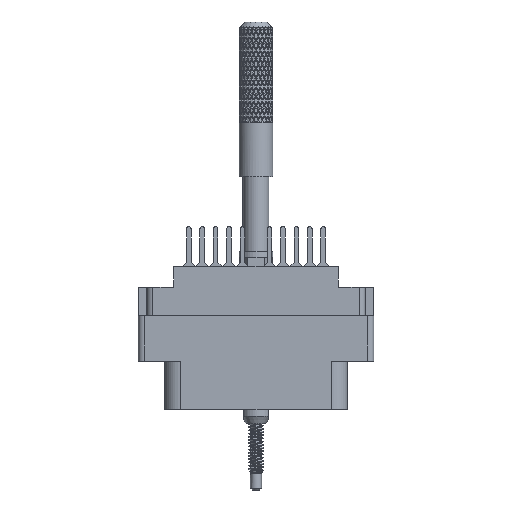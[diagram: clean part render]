
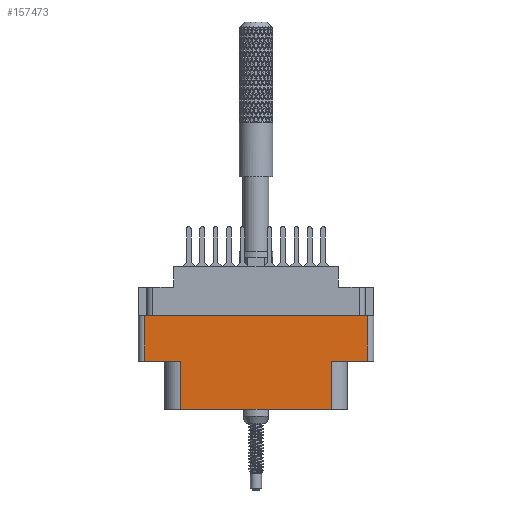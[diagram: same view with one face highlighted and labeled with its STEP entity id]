
A CAD part, front view. The second image highlights one B-rep face of the part: STEP entity #157473.
In plain terms, the highlighted planar face has unit normal (0, -1, 0).
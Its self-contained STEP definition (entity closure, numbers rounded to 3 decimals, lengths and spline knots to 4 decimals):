
#1881 = CARTESIAN_POINT ( 'NONE',  ( 0., -0.343, -0.529 ) ) ;
#3658 = LINE ( 'NONE', #1881, #130490 ) ;
#9122 = CARTESIAN_POINT ( 'NONE',  ( -0.656, -0.343, -0.798 ) ) ;
#9494 = LINE ( 'NONE', #136040, #165769 ) ;
#14220 = LINE ( 'NONE', #177238, #127639 ) ;
#16859 = ORIENTED_EDGE ( 'NONE', *, *, #94489, .T. ) ;
#19193 = EDGE_CURVE ( 'NONE', #113057, #141740, #3658, .T. ) ;
#19745 = CARTESIAN_POINT ( 'NONE',  ( -0.4205, -0.343, -0.798 ) ) ;
#21551 = ORIENTED_EDGE ( 'NONE', *, *, #19193, .F. ) ;
#22497 = CARTESIAN_POINT ( 'NONE',  ( -0.624, -0.343, -0.274 ) ) ;
#24329 = DIRECTION ( 'NONE',  ( 0., 0., -1. ) ) ;
#25174 = CARTESIAN_POINT ( 'NONE',  ( 0.4205, -0.343, -0.529 ) ) ;
#26134 = LINE ( 'NONE', #150712, #37382 ) ;
#28182 = DIRECTION ( 'NONE',  ( 1., 0., 0. ) ) ;
#31540 = EDGE_CURVE ( 'NONE', #138712, #152731, #26134, .T. ) ;
#34673 = DIRECTION ( 'NONE',  ( 1., 0., 0. ) ) ;
#36515 = VECTOR ( 'NONE', #28182, 39.3701 ) ;
#37382 = VECTOR ( 'NONE', #105849, 39.3701 ) ;
#37632 = VERTEX_POINT ( 'NONE', #130890 ) ;
#40398 = LINE ( 'NONE', #182762, #153810 ) ;
#48105 = VERTEX_POINT ( 'NONE', #68796 ) ;
#52549 = DIRECTION ( 'NONE',  ( 0., 0., 1. ) ) ;
#57459 = LINE ( 'NONE', #115490, #143591 ) ;
#58088 = DIRECTION ( 'NONE',  ( 0., 0., -1. ) ) ;
#60278 = VECTOR ( 'NONE', #52549, 39.3701 ) ;
#63743 = CARTESIAN_POINT ( 'NONE',  ( 0.624, -0.343, -0.274 ) ) ;
#67475 = DIRECTION ( 'NONE',  ( 0., -1., 0. ) ) ;
#68796 = CARTESIAN_POINT ( 'NONE',  ( 0.4205, -0.343, -0.798 ) ) ;
#71925 = ORIENTED_EDGE ( 'NONE', *, *, #114948, .T. ) ;
#73139 = EDGE_CURVE ( 'NONE', #152731, #37632, #75207, .T. ) ;
#74590 = ORIENTED_EDGE ( 'NONE', *, *, #175063, .T. ) ;
#75143 = ORIENTED_EDGE ( 'NONE', *, *, #117108, .F. ) ;
#75207 = LINE ( 'NONE', #102391, #36515 ) ;
#76199 = LINE ( 'NONE', #112153, #60278 ) ;
#81709 = VERTEX_POINT ( 'NONE', #63743 ) ;
#82576 = FACE_OUTER_BOUND ( 'NONE', #109421, .T. ) ;
#86881 = DIRECTION ( 'NONE',  ( -1., 0., 0. ) ) ;
#94489 = EDGE_CURVE ( 'NONE', #142063, #48105, #40398, .T. ) ;
#102391 = CARTESIAN_POINT ( 'NONE',  ( 0., -0.343, -0.529 ) ) ;
#105309 = ORIENTED_EDGE ( 'NONE', *, *, #73139, .T. ) ;
#105849 = DIRECTION ( 'NONE',  ( 0., 0., -1. ) ) ;
#109421 = EDGE_LOOP ( 'NONE', ( #75143, #126538, #105309, #71925, #16859, #113337, #21551, #74590 ) ) ;
#112153 = CARTESIAN_POINT ( 'NONE',  ( 0.4205, -0.343, -0.529 ) ) ;
#113057 = VERTEX_POINT ( 'NONE', #121428 ) ;
#113337 = ORIENTED_EDGE ( 'NONE', *, *, #127211, .T. ) ;
#114948 = EDGE_CURVE ( 'NONE', #37632, #142063, #14220, .T. ) ;
#115490 = CARTESIAN_POINT ( 'NONE',  ( 0.624, -0.343, -0.798 ) ) ;
#117108 = EDGE_CURVE ( 'NONE', #138712, #81709, #9494, .T. ) ;
#121428 = CARTESIAN_POINT ( 'NONE',  ( 0.624, -0.343, -0.529 ) ) ;
#125659 = PLANE ( 'NONE',  #184374 ) ;
#126538 = ORIENTED_EDGE ( 'NONE', *, *, #31540, .T. ) ;
#127211 = EDGE_CURVE ( 'NONE', #48105, #141740, #76199, .T. ) ;
#127639 = VECTOR ( 'NONE', #58088, 39.3701 ) ;
#128071 = DIRECTION ( 'NONE',  ( 1., 0., 0. ) ) ;
#130490 = VECTOR ( 'NONE', #86881, 39.3701 ) ;
#130890 = CARTESIAN_POINT ( 'NONE',  ( -0.4205, -0.343, -0.529 ) ) ;
#136040 = CARTESIAN_POINT ( 'NONE',  ( 0., -0.343, -0.274 ) ) ;
#138712 = VERTEX_POINT ( 'NONE', #22497 ) ;
#141740 = VERTEX_POINT ( 'NONE', #25174 ) ;
#142063 = VERTEX_POINT ( 'NONE', #19745 ) ;
#143591 = VECTOR ( 'NONE', #145784, 39.3701 ) ;
#145784 = DIRECTION ( 'NONE',  ( 0., 0., 1. ) ) ;
#150712 = CARTESIAN_POINT ( 'NONE',  ( -0.624, -0.343, -0.798 ) ) ;
#152731 = VERTEX_POINT ( 'NONE', #178137 ) ;
#153810 = VECTOR ( 'NONE', #128071, 39.3701 ) ;
#157473 = ADVANCED_FACE ( 'NONE', ( #82576 ), #125659, .T. ) ;
#165769 = VECTOR ( 'NONE', #34673, 39.3701 ) ;
#175063 = EDGE_CURVE ( 'NONE', #113057, #81709, #57459, .T. ) ;
#177238 = CARTESIAN_POINT ( 'NONE',  ( -0.4205, -0.343, -0.798 ) ) ;
#178137 = CARTESIAN_POINT ( 'NONE',  ( -0.624, -0.343, -0.529 ) ) ;
#182762 = CARTESIAN_POINT ( 'NONE',  ( -0.656, -0.343, -0.798 ) ) ;
#184374 = AXIS2_PLACEMENT_3D ( 'NONE', #9122, #67475, #24329 ) ;
